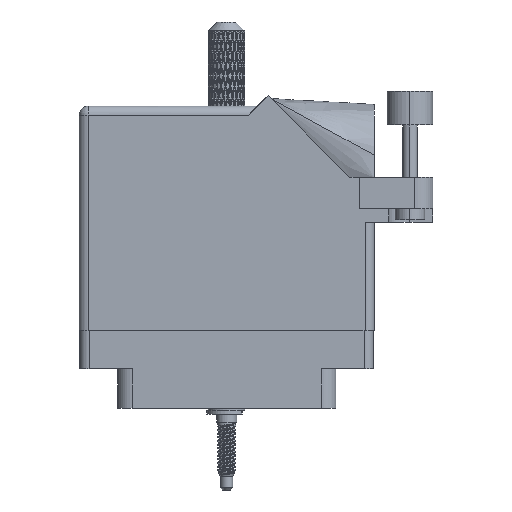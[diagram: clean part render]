
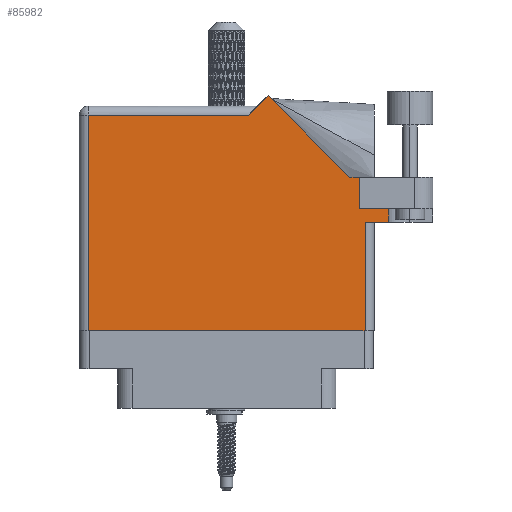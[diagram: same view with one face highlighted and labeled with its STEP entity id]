
A CAD part, front view. The second image highlights one B-rep face of the part: STEP entity #85982.
In plain terms, the highlighted face is planar.
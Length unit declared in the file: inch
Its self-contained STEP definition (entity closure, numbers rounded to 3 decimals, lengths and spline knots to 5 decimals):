
#462 = CARTESIAN_POINT ( 'NONE',  ( 1.948, 0.737, 0. ) ) ;
#1057 = CARTESIAN_POINT ( 'NONE',  ( 1.155, 1.468, 0. ) ) ;
#1575 = ORIENTED_EDGE ( 'NONE', *, *, #73074, .T. ) ;
#6214 = VERTEX_POINT ( 'NONE', #6375 ) ;
#6375 = CARTESIAN_POINT ( 'NONE',  ( 0.062, 0., 0. ) ) ;
#7461 = DIRECTION ( 'NONE',  ( 1., 0., 0. ) ) ;
#9512 = CARTESIAN_POINT ( 'NONE',  ( 0., 1.53, 0. ) ) ;
#9589 = ORIENTED_EDGE ( 'NONE', *, *, #66619, .T. ) ;
#10466 = ORIENTED_EDGE ( 'NONE', *, *, #94929, .T. ) ;
#12420 = DIRECTION ( 'NONE',  ( -0.707, -0.707, 0. ) ) ;
#12532 = FACE_OUTER_BOUND ( 'NONE', #48673, .T. ) ;
#13460 = VECTOR ( 'NONE', #7461, 39.37008 ) ;
#16538 = DIRECTION ( 'NONE',  ( 0., -1., 0. ) ) ;
#19175 = LINE ( 'NONE', #104786, #30575 ) ;
#19774 = DIRECTION ( 'NONE',  ( -1., 0., 0. ) ) ;
#19914 = CARTESIAN_POINT ( 'NONE',  ( 0., 1.468, 0. ) ) ;
#20191 = VECTOR ( 'NONE', #89595, 39.37008 ) ;
#21003 = LINE ( 'NONE', #57694, #90766 ) ;
#21776 = LINE ( 'NONE', #38443, #62307 ) ;
#24777 = CARTESIAN_POINT ( 'NONE',  ( 1.84442, 1.044, 0. ) ) ;
#25727 = VERTEX_POINT ( 'NONE', #99838 ) ;
#26801 = CARTESIAN_POINT ( 'NONE',  ( 1.84442, 1.044, 0. ) ) ;
#28262 = VECTOR ( 'NONE', #12420, 39.37008 ) ;
#28339 = LINE ( 'NONE', #462, #57520 ) ;
#28419 = CARTESIAN_POINT ( 'NONE',  ( 1.217, 1.53, 0. ) ) ;
#29575 = ORIENTED_EDGE ( 'NONE', *, *, #54223, .T. ) ;
#30575 = VECTOR ( 'NONE', #16538, 39.37008 ) ;
#31268 = VERTEX_POINT ( 'NONE', #38765 ) ;
#34628 = VECTOR ( 'NONE', #60264, 39.37008 ) ;
#36495 = CARTESIAN_POINT ( 'NONE',  ( 1.91, 1.044, 0. ) ) ;
#38021 = CARTESIAN_POINT ( 'NONE',  ( 1.91, 0.831, 0. ) ) ;
#38443 = CARTESIAN_POINT ( 'NONE',  ( 2.1115, 1.16177, 0. ) ) ;
#38765 = CARTESIAN_POINT ( 'NONE',  ( 2.1115, 0.831, 0. ) ) ;
#46172 = ORIENTED_EDGE ( 'NONE', *, *, #85904, .T. ) ;
#48040 = DIRECTION ( 'NONE',  ( 0., 1., 0. ) ) ;
#48673 = EDGE_LOOP ( 'NONE', ( #9589, #52163, #1575, #51180, #81474, #91576, #29575, #46172, #82258, #10466, #81189 ) ) ;
#48780 = EDGE_CURVE ( 'NONE', #104106, #50522, #21003, .T. ) ;
#49172 = DIRECTION ( 'NONE',  ( 0., 1., 0. ) ) ;
#50126 = CARTESIAN_POINT ( 'NONE',  ( 0., 0., 0. ) ) ;
#50522 = VERTEX_POINT ( 'NONE', #36495 ) ;
#51180 = ORIENTED_EDGE ( 'NONE', *, *, #59060, .F. ) ;
#52163 = ORIENTED_EDGE ( 'NONE', *, *, #82252, .T. ) ;
#52701 = VECTOR ( 'NONE', #71082, 39.37008 ) ;
#54223 = EDGE_CURVE ( 'NONE', #50522, #76157, #103457, .T. ) ;
#55090 = CARTESIAN_POINT ( 'NONE',  ( 1.28771, 1.60071, 0. ) ) ;
#57520 = VECTOR ( 'NONE', #48040, 39.37008 ) ;
#57694 = CARTESIAN_POINT ( 'NONE',  ( 1.91, 0.831, 0. ) ) ;
#58303 = EDGE_CURVE ( 'NONE', #84624, #69309, #84039, .T. ) ;
#59060 = EDGE_CURVE ( 'NONE', #31268, #72433, #21776, .T. ) ;
#60171 = DIRECTION ( 'NONE',  ( 0., 0., -1. ) ) ;
#60264 = DIRECTION ( 'NONE',  ( 1., 0., 0. ) ) ;
#62307 = VECTOR ( 'NONE', #96541, 39.37008 ) ;
#65512 = VERTEX_POINT ( 'NONE', #67380 ) ;
#66029 = VECTOR ( 'NONE', #69182, 39.37008 ) ;
#66488 = DIRECTION ( 'NONE',  ( 1., 0., 0. ) ) ;
#66619 = EDGE_CURVE ( 'NONE', #6214, #25727, #70783, .T. ) ;
#67380 = CARTESIAN_POINT ( 'NONE',  ( 0.062, 1.468, 0. ) ) ;
#67783 = AXIS2_PLACEMENT_3D ( 'NONE', #9512, #60171, #19774 ) ;
#69182 = DIRECTION ( 'NONE',  ( -1., 0., 0. ) ) ;
#69309 = VERTEX_POINT ( 'NONE', #1057 ) ;
#70783 = LINE ( 'NONE', #50126, #84557 ) ;
#71082 = DIRECTION ( 'NONE',  ( -1., 0., 0. ) ) ;
#72433 = VERTEX_POINT ( 'NONE', #77443 ) ;
#73074 = EDGE_CURVE ( 'NONE', #85728, #72433, #86989, .T. ) ;
#74365 = PLANE ( 'NONE',  #67783 ) ;
#75218 = LINE ( 'NONE', #100931, #34628 ) ;
#76157 = VERTEX_POINT ( 'NONE', #26801 ) ;
#76900 = CARTESIAN_POINT ( 'NONE',  ( 1.948, 0.737, 0. ) ) ;
#77443 = CARTESIAN_POINT ( 'NONE',  ( 2.1115, 0.737, 0. ) ) ;
#81189 = ORIENTED_EDGE ( 'NONE', *, *, #84349, .T. ) ;
#81474 = ORIENTED_EDGE ( 'NONE', *, *, #82658, .F. ) ;
#82252 = EDGE_CURVE ( 'NONE', #25727, #85728, #28339, .T. ) ;
#82258 = ORIENTED_EDGE ( 'NONE', *, *, #58303, .T. ) ;
#82658 = EDGE_CURVE ( 'NONE', #104106, #31268, #75218, .T. ) ;
#84039 = LINE ( 'NONE', #28419, #28262 ) ;
#84349 = EDGE_CURVE ( 'NONE', #65512, #6214, #19175, .T. ) ;
#84557 = VECTOR ( 'NONE', #66488, 39.37008 ) ;
#84624 = VERTEX_POINT ( 'NONE', #55090 ) ;
#85728 = VERTEX_POINT ( 'NONE', #76900 ) ;
#85904 = EDGE_CURVE ( 'NONE', #76157, #84624, #101275, .T. ) ;
#85982 = ADVANCED_FACE ( 'NONE', ( #12532 ), #74365, .F. ) ;
#86989 = LINE ( 'NONE', #96050, #13460 ) ;
#89595 = DIRECTION ( 'NONE',  ( -0.707, 0.707, 0. ) ) ;
#90104 = LINE ( 'NONE', #19914, #66029 ) ;
#90766 = VECTOR ( 'NONE', #49172, 39.37008 ) ;
#91576 = ORIENTED_EDGE ( 'NONE', *, *, #48780, .T. ) ;
#94929 = EDGE_CURVE ( 'NONE', #69309, #65512, #90104, .T. ) ;
#96050 = CARTESIAN_POINT ( 'NONE',  ( 2.01, 0.737, 0. ) ) ;
#96541 = DIRECTION ( 'NONE',  ( 0., -1., 0. ) ) ;
#99838 = CARTESIAN_POINT ( 'NONE',  ( 1.948, 0., 0. ) ) ;
#100931 = CARTESIAN_POINT ( 'NONE',  ( 1.91, 0.831, 0. ) ) ;
#101275 = LINE ( 'NONE', #24777, #20191 ) ;
#103304 = CARTESIAN_POINT ( 'NONE',  ( 2.41, 1.044, 0. ) ) ;
#103457 = LINE ( 'NONE', #103304, #52701 ) ;
#104106 = VERTEX_POINT ( 'NONE', #38021 ) ;
#104786 = CARTESIAN_POINT ( 'NONE',  ( 0.062, 0., 0. ) ) ;
